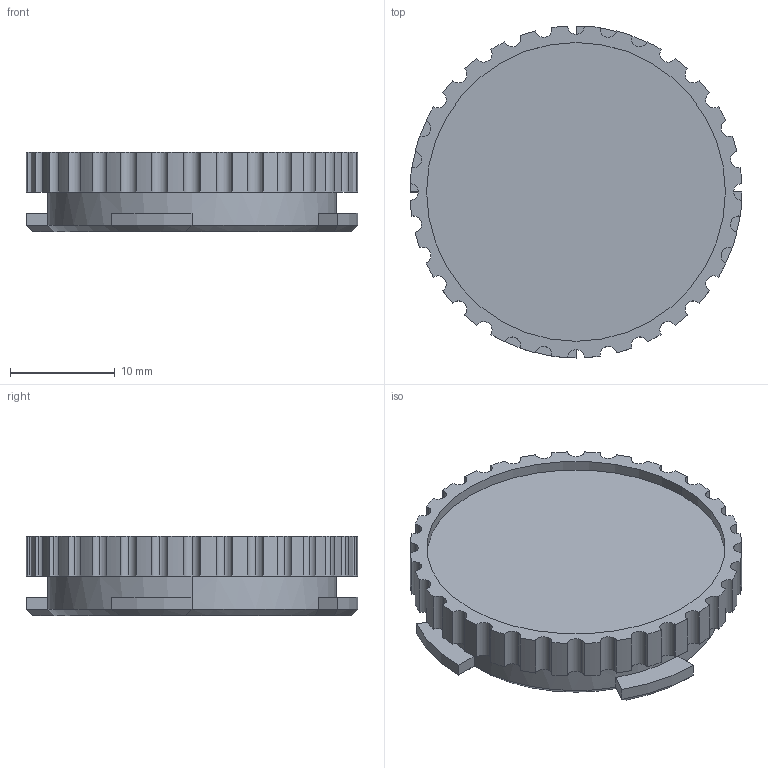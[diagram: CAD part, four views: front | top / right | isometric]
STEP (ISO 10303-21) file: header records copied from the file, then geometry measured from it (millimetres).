
FILE_DESCRIPTION (( 'STEP AP203' ), '1' );
FILE_NAME ('AF-HF-TK-PRT-002-STEP.STEP', '2020-12-04T13:13:54', ( '' ), ( '' ), 'SwSTEP 2.0', 'SolidWorks 2018', '' );
FILE_SCHEMA (( 'CONFIG_CONTROL_DESIGN' ));
Length unit declared in the file: inch
Products named in the file (1): AF-HF-TK-PRT-002-STEP
Bounding box: 31.75 x 31.75 x 7.62 mm (x, y, z)
Volume: 3660.5 mm3; surface area: 2636.4 mm2
Topology: 1 solids, 1 shells, 128 faces, 345 edges, 222 vertices
Faces by surface type: cylinder 89, plane 24, cone 13, sphere 2
Entity records: 4191 total; most frequent: DIRECTION 786, CARTESIAN_POINT 744, ORIENTED_EDGE 690, EDGE_CURVE 345, AXIS2_PLACEMENT_3D 328, VERTEX_POINT 222, CIRCLE 199, EDGE_LOOP 131
